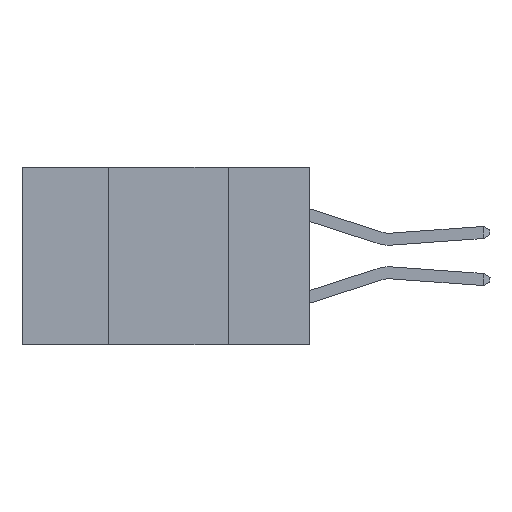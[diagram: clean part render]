
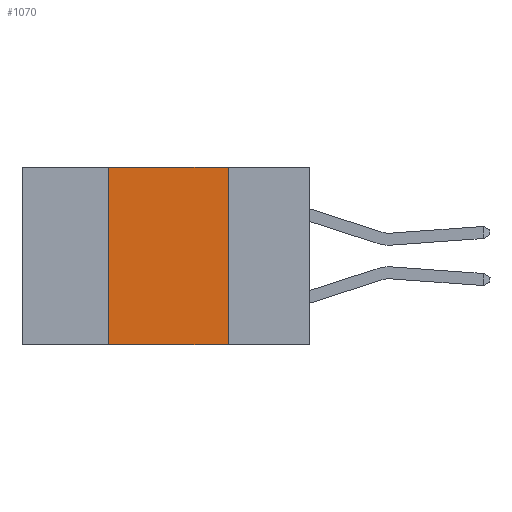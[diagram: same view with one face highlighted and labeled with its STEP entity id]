
A CAD part, left-side view. The second image highlights one B-rep face of the part: STEP entity #1070.
In plain terms, the highlighted planar face has unit normal (-1, 0, 0).
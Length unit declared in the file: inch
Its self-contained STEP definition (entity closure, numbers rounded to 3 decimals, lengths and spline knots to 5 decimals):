
#1070 = ADVANCED_FACE ( 'NONE', ( #2138 ), #14866, .F. ) ;
#1188 = VERTEX_POINT ( 'NONE', #6735 ) ;
#1422 = CARTESIAN_POINT ( 'NONE',  ( 0., 0.42, 0. ) ) ;
#1985 = DIRECTION ( 'NONE',  ( 0., 0., -1. ) ) ;
#2138 = FACE_OUTER_BOUND ( 'NONE', #10111, .T. ) ;
#2230 = ORIENTED_EDGE ( 'NONE', *, *, #5265, .F. ) ;
#2905 = LINE ( 'NONE', #8143, #5789 ) ;
#2917 = EDGE_CURVE ( 'NONE', #1188, #11803, #2905, .T. ) ;
#3726 = CARTESIAN_POINT ( 'NONE',  ( 0., 0.6, 0. ) ) ;
#3762 = LINE ( 'NONE', #5437, #4948 ) ;
#3786 = DIRECTION ( 'NONE',  ( 0., 0., -1. ) ) ;
#4257 = ORIENTED_EDGE ( 'NONE', *, *, #10221, .F. ) ;
#4553 = VECTOR ( 'NONE', #13684, 39.37008 ) ;
#4874 = AXIS2_PLACEMENT_3D ( 'NONE', #3726, #7529, #3786 ) ;
#4948 = VECTOR ( 'NONE', #13904, 39.37008 ) ;
#5199 = ORIENTED_EDGE ( 'NONE', *, *, #2917, .F. ) ;
#5265 = EDGE_CURVE ( 'NONE', #11056, #1188, #3762, .T. ) ;
#5437 = CARTESIAN_POINT ( 'NONE',  ( 0., 0.6, 0. ) ) ;
#5567 = VECTOR ( 'NONE', #6388, 39.37008 ) ;
#5789 = VECTOR ( 'NONE', #1985, 39.37008 ) ;
#6388 = DIRECTION ( 'NONE',  ( 0., -1., 0. ) ) ;
#6684 = CARTESIAN_POINT ( 'NONE',  ( 0., 0.42, 0. ) ) ;
#6735 = CARTESIAN_POINT ( 'NONE',  ( 0., 0.17, 0. ) ) ;
#6921 = LINE ( 'NONE', #8768, #5567 ) ;
#6932 = ORIENTED_EDGE ( 'NONE', *, *, #9560, .T. ) ;
#7529 = DIRECTION ( 'NONE',  ( 1., 0., 0. ) ) ;
#8143 = CARTESIAN_POINT ( 'NONE',  ( 0., 0.17, 0. ) ) ;
#8487 = CARTESIAN_POINT ( 'NONE',  ( 0., 0.42, -0.37 ) ) ;
#8768 = CARTESIAN_POINT ( 'NONE',  ( 0., 0.6, -0.37 ) ) ;
#8773 = LINE ( 'NONE', #1422, #4553 ) ;
#9560 = EDGE_CURVE ( 'NONE', #13577, #11803, #6921, .T. ) ;
#10111 = EDGE_LOOP ( 'NONE', ( #5199, #2230, #4257, #6932 ) ) ;
#10221 = EDGE_CURVE ( 'NONE', #13577, #11056, #8773, .T. ) ;
#11056 = VERTEX_POINT ( 'NONE', #6684 ) ;
#11803 = VERTEX_POINT ( 'NONE', #14092 ) ;
#13577 = VERTEX_POINT ( 'NONE', #8487 ) ;
#13684 = DIRECTION ( 'NONE',  ( 0., 0., 1. ) ) ;
#13904 = DIRECTION ( 'NONE',  ( 0., -1., 0. ) ) ;
#14092 = CARTESIAN_POINT ( 'NONE',  ( 0., 0.17, -0.37 ) ) ;
#14866 = PLANE ( 'NONE',  #4874 ) ;
